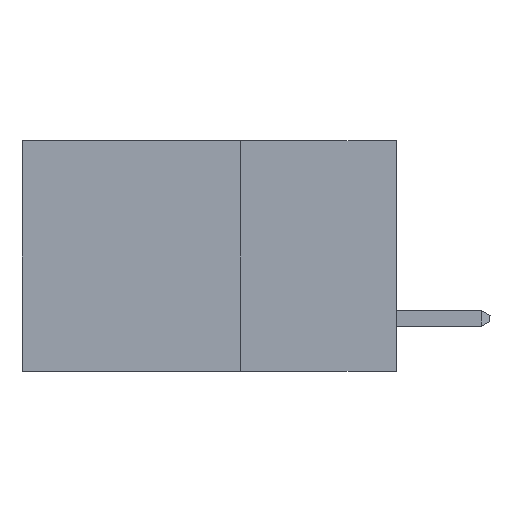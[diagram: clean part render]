
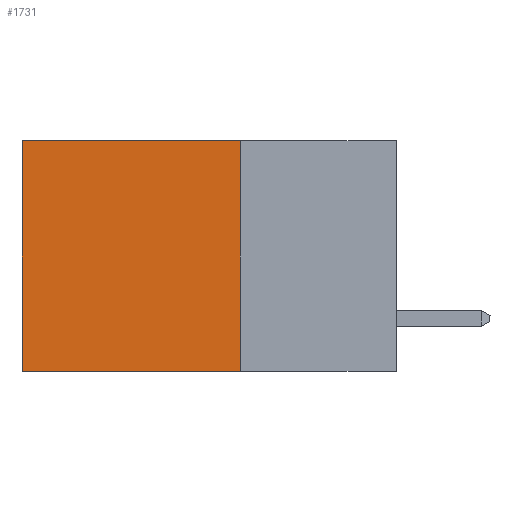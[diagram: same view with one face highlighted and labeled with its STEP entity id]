
A CAD part, left-side view. The second image highlights one B-rep face of the part: STEP entity #1731.
In plain terms, the highlighted planar face has unit normal (-1, 0, 0).
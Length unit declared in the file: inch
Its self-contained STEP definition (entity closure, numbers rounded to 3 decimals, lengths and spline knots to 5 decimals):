
#96 = VERTEX_POINT ( 'NONE', #4988 ) ;
#163 = CARTESIAN_POINT ( 'NONE',  ( 0.2615, 0.6, -0.37 ) ) ;
#402 = DIRECTION ( 'NONE',  ( 0., 0., -1. ) ) ;
#628 = VECTOR ( 'NONE', #2412, 39.37008 ) ;
#806 = DIRECTION ( 'NONE',  ( 0., 1., 0. ) ) ;
#960 = CARTESIAN_POINT ( 'NONE',  ( 0.2615, 0.25, 0. ) ) ;
#1453 = VECTOR ( 'NONE', #402, 39.37008 ) ;
#1731 = ADVANCED_FACE ( 'NONE', ( #9907 ), #10440, .F. ) ;
#2412 = DIRECTION ( 'NONE',  ( 0., 1., 0. ) ) ;
#2510 = VERTEX_POINT ( 'NONE', #163 ) ;
#2716 = EDGE_CURVE ( 'NONE', #7799, #8590, #8196, .T. ) ;
#3009 = EDGE_CURVE ( 'NONE', #96, #2510, #3958, .T. ) ;
#3638 = CARTESIAN_POINT ( 'NONE',  ( 0.2615, 0.25, -0.37 ) ) ;
#3958 = LINE ( 'NONE', #8437, #628 ) ;
#4786 = LINE ( 'NONE', #11558, #1453 ) ;
#4829 = ORIENTED_EDGE ( 'NONE', *, *, #8138, .T. ) ;
#4950 = VECTOR ( 'NONE', #806, 39.37008 ) ;
#4987 = ORIENTED_EDGE ( 'NONE', *, *, #3009, .F. ) ;
#4988 = CARTESIAN_POINT ( 'NONE',  ( 0.2615, 0.25, -0.37 ) ) ;
#5857 = DIRECTION ( 'NONE',  ( 0., 0., -1. ) ) ;
#5894 = DIRECTION ( 'NONE',  ( 1., 0., 0. ) ) ;
#6055 = ORIENTED_EDGE ( 'NONE', *, *, #2716, .T. ) ;
#6191 = ORIENTED_EDGE ( 'NONE', *, *, #10664, .F. ) ;
#6783 = CARTESIAN_POINT ( 'NONE',  ( 0.2615, 0.25, 0. ) ) ;
#7799 = VERTEX_POINT ( 'NONE', #960 ) ;
#7813 = VECTOR ( 'NONE', #9513, 39.37008 ) ;
#8138 = EDGE_CURVE ( 'NONE', #8590, #2510, #4786, .T. ) ;
#8196 = LINE ( 'NONE', #6783, #4950 ) ;
#8437 = CARTESIAN_POINT ( 'NONE',  ( 0.2615, 0.25, -0.37 ) ) ;
#8590 = VERTEX_POINT ( 'NONE', #14806 ) ;
#9513 = DIRECTION ( 'NONE',  ( 0., 0., -1. ) ) ;
#9907 = FACE_OUTER_BOUND ( 'NONE', #13197, .T. ) ;
#10440 = PLANE ( 'NONE',  #13743 ) ;
#10664 = EDGE_CURVE ( 'NONE', #7799, #96, #14494, .T. ) ;
#11558 = CARTESIAN_POINT ( 'NONE',  ( 0.2615, 0.6, -0.37 ) ) ;
#13197 = EDGE_LOOP ( 'NONE', ( #4829, #4987, #6191, #6055 ) ) ;
#13743 = AXIS2_PLACEMENT_3D ( 'NONE', #3638, #5894, #5857 ) ;
#14455 = CARTESIAN_POINT ( 'NONE',  ( 0.2615, 0.25, -0.37 ) ) ;
#14494 = LINE ( 'NONE', #14455, #7813 ) ;
#14806 = CARTESIAN_POINT ( 'NONE',  ( 0.2615, 0.6, 0. ) ) ;
